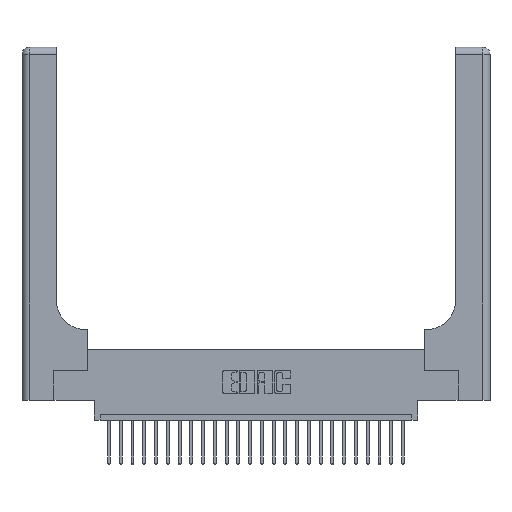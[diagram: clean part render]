
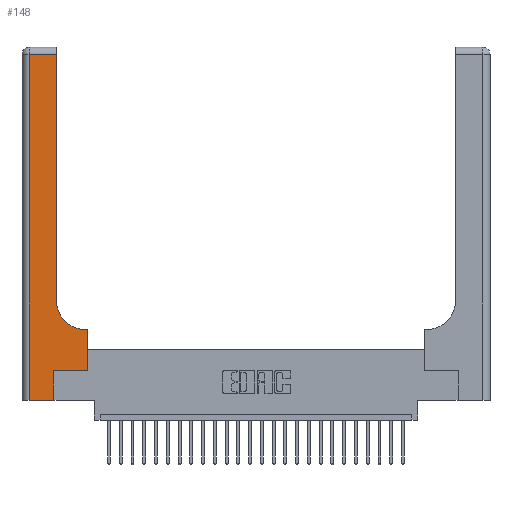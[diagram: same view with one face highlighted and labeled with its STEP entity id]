
A CAD part, top view. The second image highlights one B-rep face of the part: STEP entity #148.
In plain terms, the highlighted planar face has unit normal (0, 0, 1).
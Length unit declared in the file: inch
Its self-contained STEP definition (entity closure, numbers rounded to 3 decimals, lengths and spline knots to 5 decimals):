
#148 = ADVANCED_FACE ( 'NONE', ( #6414 ), #26776, .F. ) ;
#492 = ORIENTED_EDGE ( 'NONE', *, *, #12558, .T. ) ;
#741 = CARTESIAN_POINT ( 'NONE',  ( 0.5585, 0.25, 0.37 ) ) ;
#1108 = EDGE_CURVE ( 'NONE', #1203, #7907, #13581, .T. ) ;
#1203 = VERTEX_POINT ( 'NONE', #21088 ) ;
#1288 = ORIENTED_EDGE ( 'NONE', *, *, #2022, .T. ) ;
#2022 = EDGE_CURVE ( 'NONE', #12733, #1203, #23976, .T. ) ;
#2330 = EDGE_CURVE ( 'NONE', #7907, #15165, #20080, .T. ) ;
#2384 = DIRECTION ( 'NONE',  ( 0., 0., -1. ) ) ;
#3378 = CARTESIAN_POINT ( 'NONE',  ( 0.5585, 0.6, 0.37 ) ) ;
#3410 = LINE ( 'NONE', #15069, #10616 ) ;
#4257 = DIRECTION ( 'NONE',  ( 0., -1., 0. ) ) ;
#4595 = CARTESIAN_POINT ( 'NONE',  ( 0., 2.94, 0.37 ) ) ;
#4731 = VERTEX_POINT ( 'NONE', #16529 ) ;
#5083 = ORIENTED_EDGE ( 'NONE', *, *, #2330, .T. ) ;
#5107 = ORIENTED_EDGE ( 'NONE', *, *, #22086, .T. ) ;
#5970 = CARTESIAN_POINT ( 'NONE',  ( 0.2915, 0.6, 0.37 ) ) ;
#6182 = CARTESIAN_POINT ( 'NONE',  ( 0.2915, 3., 0.37 ) ) ;
#6387 = EDGE_CURVE ( 'NONE', #15165, #4731, #11383, .T. ) ;
#6414 = FACE_OUTER_BOUND ( 'NONE', #10841, .T. ) ;
#6620 = VECTOR ( 'NONE', #17521, 39.37008 ) ;
#6855 = VERTEX_POINT ( 'NONE', #3378 ) ;
#6965 = DIRECTION ( 'NONE',  ( 0., 0., -1. ) ) ;
#7304 = DIRECTION ( 'NONE',  ( 0., 1., 0. ) ) ;
#7683 = VECTOR ( 'NONE', #26979, 39.37008 ) ;
#7907 = VERTEX_POINT ( 'NONE', #10728 ) ;
#8005 = CARTESIAN_POINT ( 'NONE',  ( 0.269, 0., 0.37 ) ) ;
#8870 = CARTESIAN_POINT ( 'NONE',  ( 0., 0., 0.37 ) ) ;
#8895 = LINE ( 'NONE', #5970, #23221 ) ;
#9058 = VERTEX_POINT ( 'NONE', #741 ) ;
#10061 = VECTOR ( 'NONE', #7304, 39.37008 ) ;
#10365 = ORIENTED_EDGE ( 'NONE', *, *, #1108, .T. ) ;
#10457 = DIRECTION ( 'NONE',  ( -1., 0., 0. ) ) ;
#10616 = VECTOR ( 'NONE', #13626, 39.37008 ) ;
#10728 = CARTESIAN_POINT ( 'NONE',  ( 0.06, 0., 0.37 ) ) ;
#10841 = EDGE_LOOP ( 'NONE', ( #5107, #1288, #10365, #5083, #22699, #11521, #492, #23454, #19701 ) ) ;
#10853 = CARTESIAN_POINT ( 'NONE',  ( 0.06, 3., 0.37 ) ) ;
#11070 = VECTOR ( 'NONE', #4257, 39.37008 ) ;
#11304 = CARTESIAN_POINT ( 'NONE',  ( 0.5415, 0.85, 0.37 ) ) ;
#11383 = LINE ( 'NONE', #11509, #10061 ) ;
#11509 = CARTESIAN_POINT ( 'NONE',  ( 0.269, 0., 0.37 ) ) ;
#11521 = ORIENTED_EDGE ( 'NONE', *, *, #13934, .T. ) ;
#12558 = EDGE_CURVE ( 'NONE', #9058, #6855, #14439, .T. ) ;
#12733 = VERTEX_POINT ( 'NONE', #20239 ) ;
#12882 = EDGE_CURVE ( 'NONE', #6855, #17498, #8895, .T. ) ;
#13119 = EDGE_CURVE ( 'NONE', #17498, #18711, #19979, .T. ) ;
#13514 = DIRECTION ( 'NONE',  ( 1., 0., 0. ) ) ;
#13581 = LINE ( 'NONE', #10853, #11070 ) ;
#13626 = DIRECTION ( 'NONE',  ( 1., 0., 0. ) ) ;
#13934 = EDGE_CURVE ( 'NONE', #4731, #9058, #3410, .T. ) ;
#14012 = DIRECTION ( 'NONE',  ( -1., 0., 0. ) ) ;
#14439 = LINE ( 'NONE', #21709, #6620 ) ;
#15069 = CARTESIAN_POINT ( 'NONE',  ( 0.269, 0.25, 0.37 ) ) ;
#15165 = VERTEX_POINT ( 'NONE', #8005 ) ;
#16529 = CARTESIAN_POINT ( 'NONE',  ( 0.269, 0.25, 0.37 ) ) ;
#16556 = DIRECTION ( 'NONE',  ( -1., 0., 0. ) ) ;
#17498 = VERTEX_POINT ( 'NONE', #27031 ) ;
#17521 = DIRECTION ( 'NONE',  ( 0., 1., 0. ) ) ;
#17773 = CARTESIAN_POINT ( 'NONE',  ( 0.2915, 0.85, 0.37 ) ) ;
#18413 = VECTOR ( 'NONE', #14012, 39.37008 ) ;
#18474 = CARTESIAN_POINT ( 'NONE',  ( 0., 3., 0.37 ) ) ;
#18711 = VERTEX_POINT ( 'NONE', #17773 ) ;
#19408 = LINE ( 'NONE', #6182, #7683 ) ;
#19701 = ORIENTED_EDGE ( 'NONE', *, *, #13119, .T. ) ;
#19979 = CIRCLE ( 'NONE', #25861, 0.25 ) ;
#20080 = LINE ( 'NONE', #8870, #24944 ) ;
#20239 = CARTESIAN_POINT ( 'NONE',  ( 0.2915, 2.94, 0.37 ) ) ;
#21088 = CARTESIAN_POINT ( 'NONE',  ( 0.06, 2.94, 0.37 ) ) ;
#21709 = CARTESIAN_POINT ( 'NONE',  ( 0.5585, 0.25, 0.37 ) ) ;
#22086 = EDGE_CURVE ( 'NONE', #18711, #12733, #19408, .T. ) ;
#22699 = ORIENTED_EDGE ( 'NONE', *, *, #6387, .T. ) ;
#23221 = VECTOR ( 'NONE', #16556, 39.37008 ) ;
#23454 = ORIENTED_EDGE ( 'NONE', *, *, #12882, .T. ) ;
#23468 = DIRECTION ( 'NONE',  ( 1., 0., 0. ) ) ;
#23976 = LINE ( 'NONE', #4595, #18413 ) ;
#24944 = VECTOR ( 'NONE', #13514, 39.37008 ) ;
#25282 = AXIS2_PLACEMENT_3D ( 'NONE', #18474, #2384, #10457 ) ;
#25861 = AXIS2_PLACEMENT_3D ( 'NONE', #11304, #6965, #23468 ) ;
#26776 = PLANE ( 'NONE',  #25282 ) ;
#26979 = DIRECTION ( 'NONE',  ( 0., 1., 0. ) ) ;
#27031 = CARTESIAN_POINT ( 'NONE',  ( 0.5415, 0.6, 0.37 ) ) ;
